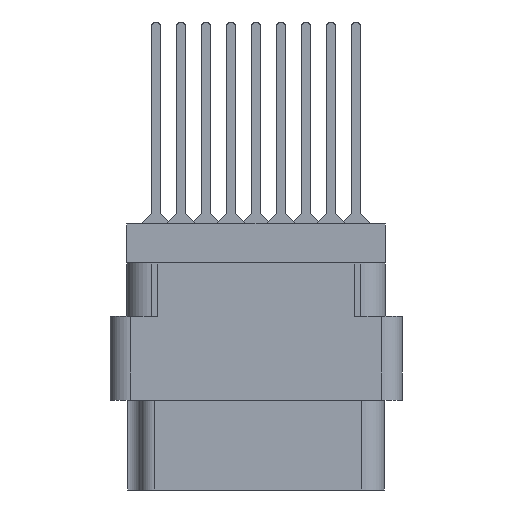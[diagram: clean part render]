
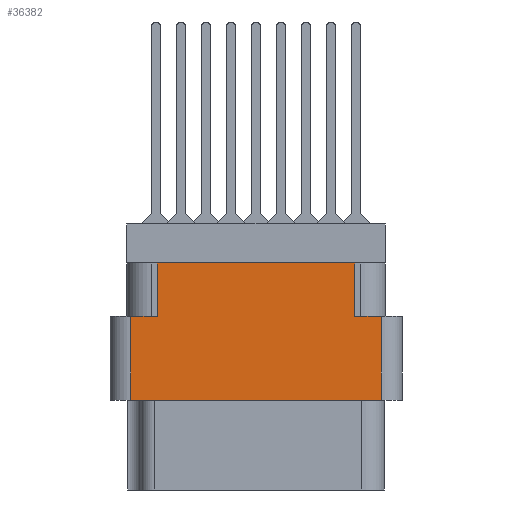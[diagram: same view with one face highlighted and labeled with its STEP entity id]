
A CAD part, left-side view. The second image highlights one B-rep face of the part: STEP entity #36382.
In plain terms, the highlighted planar face has unit normal (-1, 0, 0).
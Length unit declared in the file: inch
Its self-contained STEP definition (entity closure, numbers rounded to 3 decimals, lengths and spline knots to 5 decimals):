
#243 = VECTOR ( 'NONE', #18594, 39.37008 ) ;
#1235 = EDGE_CURVE ( 'NONE', #33983, #37965, #9464, .T. ) ;
#2439 = DIRECTION ( 'NONE',  ( 0., 0., 1. ) ) ;
#4106 = ORIENTED_EDGE ( 'NONE', *, *, #1235, .T. ) ;
#4373 = CARTESIAN_POINT ( 'NONE',  ( -1., 0., -0.529 ) ) ;
#5688 = EDGE_LOOP ( 'NONE', ( #14452, #4106, #8120, #35367, #14056, #27066, #25936, #11964 ) ) ;
#6523 = EDGE_CURVE ( 'NONE', #14434, #17135, #33413, .T. ) ;
#6984 = LINE ( 'NONE', #18517, #36901 ) ;
#7509 = VERTEX_POINT ( 'NONE', #36199 ) ;
#8120 = ORIENTED_EDGE ( 'NONE', *, *, #26371, .F. ) ;
#8744 = VERTEX_POINT ( 'NONE', #10492 ) ;
#9464 = LINE ( 'NONE', #31280, #24399 ) ;
#10492 = CARTESIAN_POINT ( 'NONE',  ( -1., -0.376, -0.529 ) ) ;
#10696 = CARTESIAN_POINT ( 'NONE',  ( -1., 0.376, -0.529 ) ) ;
#11538 = LINE ( 'NONE', #4373, #38769 ) ;
#11964 = ORIENTED_EDGE ( 'NONE', *, *, #32418, .F. ) ;
#13801 = FACE_OUTER_BOUND ( 'NONE', #5688, .T. ) ;
#13981 = VECTOR ( 'NONE', #34081, 39.37008 ) ;
#13984 = EDGE_CURVE ( 'NONE', #33983, #7509, #25590, .T. ) ;
#14056 = ORIENTED_EDGE ( 'NONE', *, *, #14728, .F. ) ;
#14434 = VERTEX_POINT ( 'NONE', #30811 ) ;
#14452 = ORIENTED_EDGE ( 'NONE', *, *, #13984, .F. ) ;
#14701 = CARTESIAN_POINT ( 'NONE',  ( -1., 0., -0.277 ) ) ;
#14728 = EDGE_CURVE ( 'NONE', #14434, #38081, #20409, .T. ) ;
#15287 = DIRECTION ( 'NONE',  ( 0., -1., 0. ) ) ;
#15534 = VECTOR ( 'NONE', #25250, 39.37008 ) ;
#16664 = VECTOR ( 'NONE', #27139, 39.37008 ) ;
#16898 = CARTESIAN_POINT ( 'NONE',  ( -1., 0.296, -0.117 ) ) ;
#17135 = VERTEX_POINT ( 'NONE', #35513 ) ;
#17606 = VECTOR ( 'NONE', #35153, 39.37008 ) ;
#18517 = CARTESIAN_POINT ( 'NONE',  ( -1., 0.438, -0.117 ) ) ;
#18594 = DIRECTION ( 'NONE',  ( 0., 0., 1. ) ) ;
#18730 = EDGE_CURVE ( 'NONE', #8744, #38081, #21914, .T. ) ;
#20046 = DIRECTION ( 'NONE',  ( -1., 0., 0. ) ) ;
#20195 = LINE ( 'NONE', #31448, #15534 ) ;
#20409 = LINE ( 'NONE', #14701, #16664 ) ;
#21489 = CARTESIAN_POINT ( 'NONE',  ( -1., -0.296, -0.277 ) ) ;
#21866 = CARTESIAN_POINT ( 'NONE',  ( -1., -0.376, -0.798 ) ) ;
#21914 = LINE ( 'NONE', #21866, #13981 ) ;
#22195 = DIRECTION ( 'NONE',  ( 0., 0., -1. ) ) ;
#24207 = CARTESIAN_POINT ( 'NONE',  ( -1., 0.376, -0.277 ) ) ;
#24399 = VECTOR ( 'NONE', #22195, 39.37008 ) ;
#25250 = DIRECTION ( 'NONE',  ( 0., 0., 1. ) ) ;
#25257 = DIRECTION ( 'NONE',  ( 0., 1., 0. ) ) ;
#25590 = LINE ( 'NONE', #32142, #17606 ) ;
#25605 = VERTEX_POINT ( 'NONE', #16898 ) ;
#25936 = ORIENTED_EDGE ( 'NONE', *, *, #34715, .F. ) ;
#26371 = EDGE_CURVE ( 'NONE', #8744, #37965, #11538, .T. ) ;
#27066 = ORIENTED_EDGE ( 'NONE', *, *, #6523, .T. ) ;
#27139 = DIRECTION ( 'NONE',  ( 0., -1., 0. ) ) ;
#29019 = PLANE ( 'NONE',  #34408 ) ;
#30811 = CARTESIAN_POINT ( 'NONE',  ( -1., -0.296, -0.277 ) ) ;
#31280 = CARTESIAN_POINT ( 'NONE',  ( -1., 0.376, -0.798 ) ) ;
#31448 = CARTESIAN_POINT ( 'NONE',  ( -1., 0.296, -0.277 ) ) ;
#32022 = CARTESIAN_POINT ( 'NONE',  ( -1., -0.438, -0.798 ) ) ;
#32142 = CARTESIAN_POINT ( 'NONE',  ( -1., 0., -0.277 ) ) ;
#32418 = EDGE_CURVE ( 'NONE', #7509, #25605, #20195, .T. ) ;
#33413 = LINE ( 'NONE', #21489, #243 ) ;
#33983 = VERTEX_POINT ( 'NONE', #24207 ) ;
#34081 = DIRECTION ( 'NONE',  ( 0., 0., 1. ) ) ;
#34408 = AXIS2_PLACEMENT_3D ( 'NONE', #32022, #20046, #2439 ) ;
#34715 = EDGE_CURVE ( 'NONE', #25605, #17135, #6984, .T. ) ;
#34794 = CARTESIAN_POINT ( 'NONE',  ( -1., -0.376, -0.277 ) ) ;
#35153 = DIRECTION ( 'NONE',  ( 0., -1., 0. ) ) ;
#35367 = ORIENTED_EDGE ( 'NONE', *, *, #18730, .T. ) ;
#35513 = CARTESIAN_POINT ( 'NONE',  ( -1., -0.296, -0.117 ) ) ;
#36199 = CARTESIAN_POINT ( 'NONE',  ( -1., 0.296, -0.277 ) ) ;
#36382 = ADVANCED_FACE ( 'NONE', ( #13801 ), #29019, .T. ) ;
#36901 = VECTOR ( 'NONE', #15287, 39.37008 ) ;
#37965 = VERTEX_POINT ( 'NONE', #10696 ) ;
#38081 = VERTEX_POINT ( 'NONE', #34794 ) ;
#38769 = VECTOR ( 'NONE', #25257, 39.37008 ) ;
